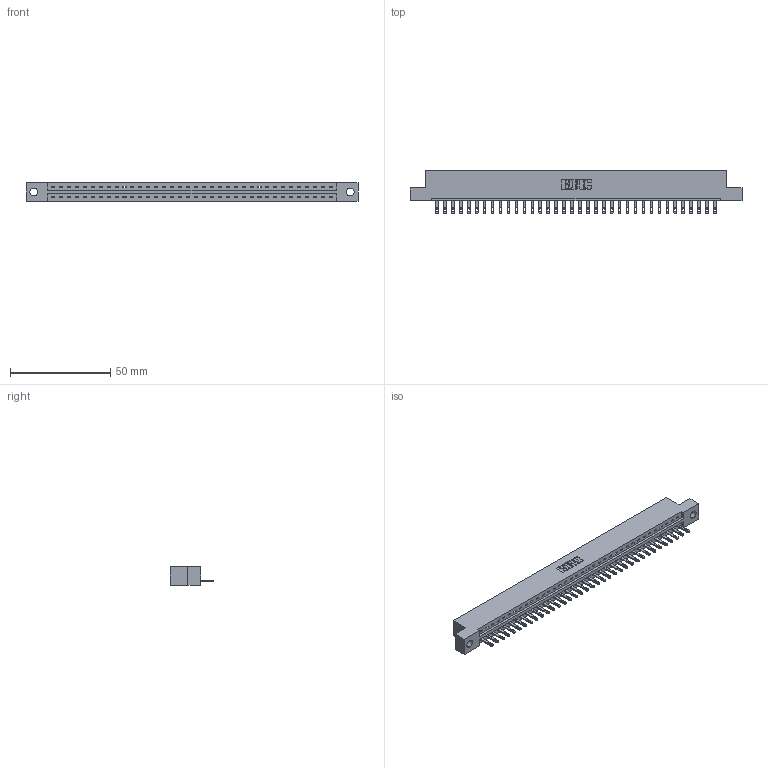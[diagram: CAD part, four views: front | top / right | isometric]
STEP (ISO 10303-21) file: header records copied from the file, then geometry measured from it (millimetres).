
FILE_DESCRIPTION (( 'STEP AP203' ), '1' );
FILE_NAME ('887-036-500-104.STEP', '2020-09-20T22:07:48', ( '' ), ( '' ), 'SwSTEP 2.0', 'SolidWorks 2020', '' );
FILE_SCHEMA (( 'CONFIG_CONTROL_DESIGN' ));
Length unit declared in the file: inch
Products named in the file (3): 887-036-500-104; 837 Part_Flush Mounting Lugs - 0.156 Dia-TH; 345-292-001_345-293-100
Assembly tree (37 placements, depth 2):
  887-036-500-104
    837 Part_Flush Mounting Lugs - 0.156 Dia-TH
    345-292-001_345-293-100  x36
Bounding box: 165.66 x 21.85 x 9.4 mm (x, y, z)
Volume: 17076.8 mm3; surface area: 17492.4 mm2
Topology: 37 solids, 37 shells, 2202 faces, 6791 edges, 4526 vertices
Faces by surface type: plane 1510, cylinder 692
Entity records: 27469 total; most frequent: CARTESIAN_POINT 4790, ORIENTED_EDGE 4762, DIRECTION 4045, EDGE_CURVE 2381, LINE 2249, VECTOR 2249, VERTEX_POINT 1586, AXIS2_PLACEMENT_3D 898
